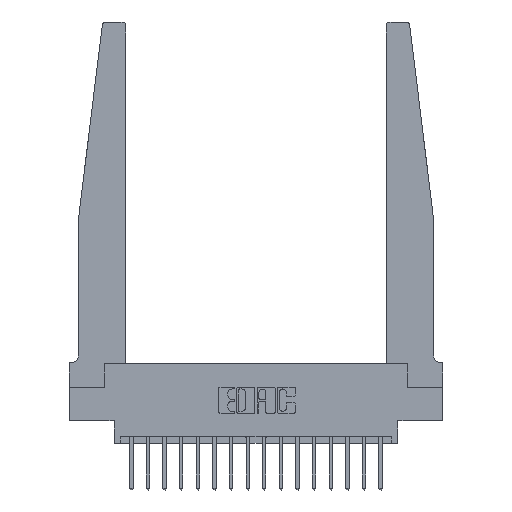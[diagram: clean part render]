
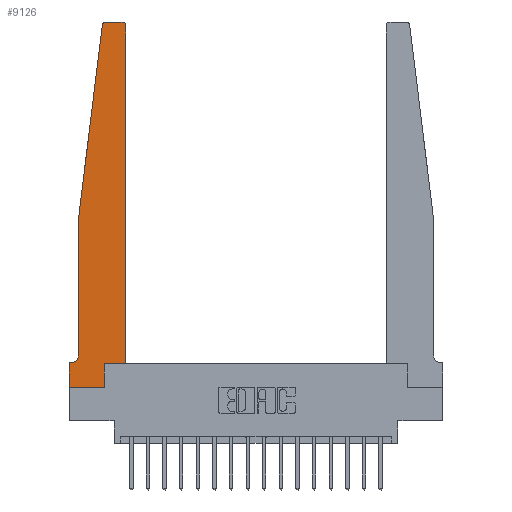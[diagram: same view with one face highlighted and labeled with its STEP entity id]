
A CAD part, top view. The second image highlights one B-rep face of the part: STEP entity #9126.
In plain terms, the highlighted planar face has unit normal (0, 0, 1).
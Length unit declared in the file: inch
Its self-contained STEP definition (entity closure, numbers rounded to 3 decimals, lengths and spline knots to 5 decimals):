
#270 = DIRECTION ( 'NONE',  ( 0., -1., 0. ) ) ;
#402 = CARTESIAN_POINT ( 'NONE',  ( 0., 0., 0.37 ) ) ;
#413 = DIRECTION ( 'NONE',  ( -1., 0., 0. ) ) ;
#519 = ORIENTED_EDGE ( 'NONE', *, *, #18151, .T. ) ;
#797 = ORIENTED_EDGE ( 'NONE', *, *, #13624, .T. ) ;
#913 = DIRECTION ( 'NONE',  ( 0., -1., 0. ) ) ;
#956 = CARTESIAN_POINT ( 'NONE',  ( 0.24675, 2.72367, 0.37 ) ) ;
#1165 = CARTESIAN_POINT ( 'NONE',  ( 0.25, 2.75, 0.37 ) ) ;
#1190 = DIRECTION ( 'NONE',  ( 0., 1., 0. ) ) ;
#1320 = EDGE_CURVE ( 'NONE', #15741, #8848, #7757, .T. ) ;
#1411 = CARTESIAN_POINT ( 'NONE',  ( 0.395, 2.72, 0.37 ) ) ;
#1460 = CARTESIAN_POINT ( 'NONE',  ( 0.425, 2.72, 0.37 ) ) ;
#1592 = ORIENTED_EDGE ( 'NONE', *, *, #11407, .T. ) ;
#1944 = CARTESIAN_POINT ( 'NONE',  ( 0.065, 1.25, 0.37 ) ) ;
#2483 = LINE ( 'NONE', #17316, #17031 ) ;
#2559 = VERTEX_POINT ( 'NONE', #3424 ) ;
#2585 = LINE ( 'NONE', #15233, #13683 ) ;
#2653 = DIRECTION ( 'NONE',  ( -1., 0., 0. ) ) ;
#2743 = VERTEX_POINT ( 'NONE', #17213 ) ;
#2826 = EDGE_CURVE ( 'NONE', #13136, #10562, #11098, .T. ) ;
#2902 = DIRECTION ( 'NONE',  ( 1., 0., 0. ) ) ;
#3411 = EDGE_CURVE ( 'NONE', #8848, #5780, #2483, .T. ) ;
#3424 = CARTESIAN_POINT ( 'NONE',  ( 0.065, 1.25, 0.37 ) ) ;
#3698 = DIRECTION ( 'NONE',  ( 1., 0., 0. ) ) ;
#3729 = CARTESIAN_POINT ( 'NONE',  ( 0.27653, 2.72, 0.37 ) ) ;
#4094 = AXIS2_PLACEMENT_3D ( 'NONE', #5820, #15971, #7280 ) ;
#4278 = VECTOR ( 'NONE', #413, 39.37008 ) ;
#4551 = CARTESIAN_POINT ( 'NONE',  ( 0.015, 0.1875, 0.37 ) ) ;
#4725 = VERTEX_POINT ( 'NONE', #15839 ) ;
#4732 = LINE ( 'NONE', #17865, #4278 ) ;
#4925 = ORIENTED_EDGE ( 'NONE', *, *, #15264, .T. ) ;
#5189 = DIRECTION ( 'NONE',  ( 1., 0., 0. ) ) ;
#5315 = CARTESIAN_POINT ( 'NONE',  ( 0.065, 0.2375, 0.37 ) ) ;
#5321 = CARTESIAN_POINT ( 'NONE',  ( 0.2605, 0.18, 0.37 ) ) ;
#5754 = CARTESIAN_POINT ( 'NONE',  ( 0.425, 0.18, 0.37 ) ) ;
#5780 = VERTEX_POINT ( 'NONE', #5321 ) ;
#5820 = CARTESIAN_POINT ( 'NONE',  ( 0., 0.1875, 0.37 ) ) ;
#5831 = DIRECTION ( 'NONE',  ( 1., 0., 0. ) ) ;
#5848 = LINE ( 'NONE', #17740, #16531 ) ;
#5864 = EDGE_CURVE ( 'NONE', #10562, #4725, #12830, .T. ) ;
#5955 = VECTOR ( 'NONE', #913, 39.37008 ) ;
#6412 = LINE ( 'NONE', #15468, #5955 ) ;
#7280 = DIRECTION ( 'NONE',  ( 1., 0., 0. ) ) ;
#7449 = CARTESIAN_POINT ( 'NONE',  ( 0.015, 0.2375, 0.37 ) ) ;
#7624 = LINE ( 'NONE', #18639, #18781 ) ;
#7757 = LINE ( 'NONE', #17479, #18472 ) ;
#8336 = AXIS2_PLACEMENT_3D ( 'NONE', #3729, #13863, #5189 ) ;
#8848 = VERTEX_POINT ( 'NONE', #17917 ) ;
#8860 = EDGE_CURVE ( 'NONE', #9572, #2559, #12520, .T. ) ;
#8891 = DIRECTION ( 'NONE',  ( -1., 0., 0. ) ) ;
#8924 = ORIENTED_EDGE ( 'NONE', *, *, #1320, .T. ) ;
#8967 = EDGE_CURVE ( 'NONE', #4725, #9572, #18018, .T. ) ;
#9005 = EDGE_CURVE ( 'NONE', #2743, #15741, #6412, .T. ) ;
#9121 = VECTOR ( 'NONE', #10567, 39.37008 ) ;
#9126 = ADVANCED_FACE ( 'NONE', ( #11828 ), #13035, .T. ) ;
#9572 = VERTEX_POINT ( 'NONE', #956 ) ;
#10024 = DIRECTION ( 'NONE',  ( 0., 1., 0. ) ) ;
#10289 = ORIENTED_EDGE ( 'NONE', *, *, #9005, .T. ) ;
#10487 = VERTEX_POINT ( 'NONE', #4551 ) ;
#10562 = VERTEX_POINT ( 'NONE', #11907 ) ;
#10567 = DIRECTION ( 'NONE',  ( -0.122, -0.992, 0. ) ) ;
#11063 = CIRCLE ( 'NONE', #17540, 0.05 ) ;
#11098 = CIRCLE ( 'NONE', #16665, 0.03 ) ;
#11407 = EDGE_CURVE ( 'NONE', #14347, #10487, #11063, .T. ) ;
#11574 = DIRECTION ( 'NONE',  ( 0., 0., 1. ) ) ;
#11828 = FACE_OUTER_BOUND ( 'NONE', #13413, .T. ) ;
#11907 = CARTESIAN_POINT ( 'NONE',  ( 0.395, 2.75, 0.37 ) ) ;
#12031 = EDGE_CURVE ( 'NONE', #2559, #14347, #5848, .T. ) ;
#12374 = VECTOR ( 'NONE', #2653, 39.37008 ) ;
#12520 = LINE ( 'NONE', #1944, #9121 ) ;
#12830 = LINE ( 'NONE', #1165, #12374 ) ;
#12981 = ORIENTED_EDGE ( 'NONE', *, *, #12031, .T. ) ;
#13035 = PLANE ( 'NONE',  #4094 ) ;
#13136 = VERTEX_POINT ( 'NONE', #1460 ) ;
#13331 = ORIENTED_EDGE ( 'NONE', *, *, #8967, .T. ) ;
#13413 = EDGE_LOOP ( 'NONE', ( #15893, #13331, #18257, #12981, #1592, #519, #10289, #8924, #16762, #4925, #797, #15908 ) ) ;
#13624 = EDGE_CURVE ( 'NONE', #14526, #13136, #7624, .T. ) ;
#13683 = VECTOR ( 'NONE', #3698, 39.37008 ) ;
#13863 = DIRECTION ( 'NONE',  ( 0., 0., 1. ) ) ;
#14347 = VERTEX_POINT ( 'NONE', #5315 ) ;
#14526 = VERTEX_POINT ( 'NONE', #5754 ) ;
#15233 = CARTESIAN_POINT ( 'NONE',  ( 0.425, 0.18, 0.37 ) ) ;
#15264 = EDGE_CURVE ( 'NONE', #5780, #14526, #2585, .T. ) ;
#15468 = CARTESIAN_POINT ( 'NONE',  ( 0., 0., 0.37 ) ) ;
#15741 = VERTEX_POINT ( 'NONE', #402 ) ;
#15839 = CARTESIAN_POINT ( 'NONE',  ( 0.27653, 2.75, 0.37 ) ) ;
#15893 = ORIENTED_EDGE ( 'NONE', *, *, #5864, .T. ) ;
#15908 = ORIENTED_EDGE ( 'NONE', *, *, #2826, .T. ) ;
#15971 = DIRECTION ( 'NONE',  ( 0., 0., 1. ) ) ;
#16531 = VECTOR ( 'NONE', #270, 39.37008 ) ;
#16665 = AXIS2_PLACEMENT_3D ( 'NONE', #1411, #11574, #2902 ) ;
#16762 = ORIENTED_EDGE ( 'NONE', *, *, #3411, .T. ) ;
#17031 = VECTOR ( 'NONE', #10024, 39.37008 ) ;
#17213 = CARTESIAN_POINT ( 'NONE',  ( 0., 0.1875, 0.37 ) ) ;
#17316 = CARTESIAN_POINT ( 'NONE',  ( 0.2605, 0.18, 0.37 ) ) ;
#17479 = CARTESIAN_POINT ( 'NONE',  ( 0., 0., 0.37 ) ) ;
#17540 = AXIS2_PLACEMENT_3D ( 'NONE', #7449, #17634, #8891 ) ;
#17634 = DIRECTION ( 'NONE',  ( 0., 0., -1. ) ) ;
#17740 = CARTESIAN_POINT ( 'NONE',  ( 0.065, 1.25, 0.37 ) ) ;
#17865 = CARTESIAN_POINT ( 'NONE',  ( 0.065, 0.1875, 0.37 ) ) ;
#17917 = CARTESIAN_POINT ( 'NONE',  ( 0.2605, 0., 0.37 ) ) ;
#18018 = CIRCLE ( 'NONE', #8336, 0.03 ) ;
#18151 = EDGE_CURVE ( 'NONE', #10487, #2743, #4732, .T. ) ;
#18257 = ORIENTED_EDGE ( 'NONE', *, *, #8860, .T. ) ;
#18472 = VECTOR ( 'NONE', #5831, 39.37008 ) ;
#18639 = CARTESIAN_POINT ( 'NONE',  ( 0.425, 0.18, 0.37 ) ) ;
#18781 = VECTOR ( 'NONE', #1190, 39.37008 ) ;
